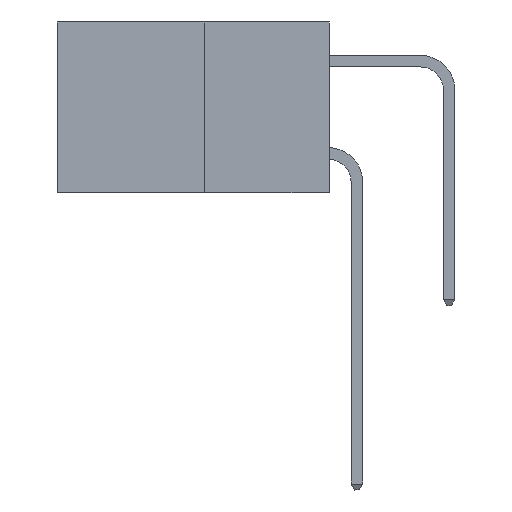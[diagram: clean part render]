
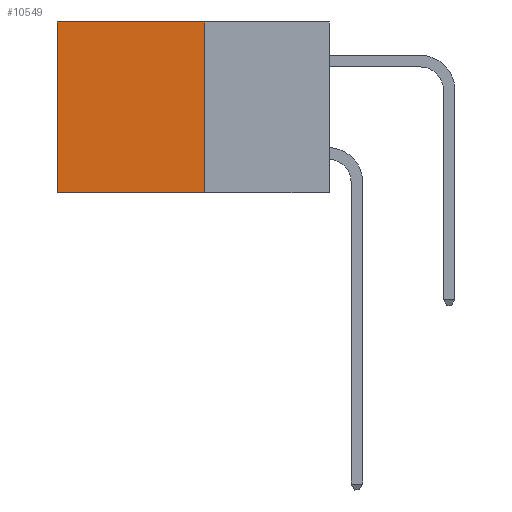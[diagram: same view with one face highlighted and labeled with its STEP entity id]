
A CAD part, left-side view. The second image highlights one B-rep face of the part: STEP entity #10549.
In plain terms, the highlighted planar face has unit normal (-1, 0, 0).
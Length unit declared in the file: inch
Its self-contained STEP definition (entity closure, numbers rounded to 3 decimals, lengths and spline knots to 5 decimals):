
#192 = AXIS2_PLACEMENT_3D ( 'NONE', #8386, #10762, #3405 ) ;
#1339 = DIRECTION ( 'NONE',  ( 0., 1., 0. ) ) ;
#1359 = ORIENTED_EDGE ( 'NONE', *, *, #1635, .T. ) ;
#1572 = CARTESIAN_POINT ( 'NONE',  ( 0.277, 0.27, -0.37 ) ) ;
#1635 = EDGE_CURVE ( 'NONE', #6401, #8254, #6325, .T. ) ;
#2506 = ORIENTED_EDGE ( 'NONE', *, *, #9012, .T. ) ;
#2577 = VECTOR ( 'NONE', #10705, 39.37008 ) ;
#3405 = DIRECTION ( 'NONE',  ( 0., 0., -1. ) ) ;
#3964 = VERTEX_POINT ( 'NONE', #10169 ) ;
#5584 = EDGE_CURVE ( 'NONE', #3964, #8254, #15202, .T. ) ;
#6325 = LINE ( 'NONE', #10808, #2577 ) ;
#6401 = VERTEX_POINT ( 'NONE', #11030 ) ;
#6973 = ORIENTED_EDGE ( 'NONE', *, *, #5584, .F. ) ;
#7156 = PLANE ( 'NONE',  #192 ) ;
#7294 = EDGE_CURVE ( 'NONE', #9734, #3964, #13034, .T. ) ;
#8116 = FACE_OUTER_BOUND ( 'NONE', #10496, .T. ) ;
#8254 = VERTEX_POINT ( 'NONE', #13641 ) ;
#8386 = CARTESIAN_POINT ( 'NONE',  ( 0.277, 0.27, -0.37 ) ) ;
#9012 = EDGE_CURVE ( 'NONE', #9734, #6401, #12447, .T. ) ;
#9734 = VERTEX_POINT ( 'NONE', #9985 ) ;
#9838 = DIRECTION ( 'NONE',  ( 0., 0., -1. ) ) ;
#9985 = CARTESIAN_POINT ( 'NONE',  ( 0.277, 0.27, 0. ) ) ;
#10169 = CARTESIAN_POINT ( 'NONE',  ( 0.277, 0.27, -0.37 ) ) ;
#10496 = EDGE_LOOP ( 'NONE', ( #1359, #6973, #11989, #2506 ) ) ;
#10549 = ADVANCED_FACE ( 'NONE', ( #8116 ), #7156, .F. ) ;
#10705 = DIRECTION ( 'NONE',  ( 0., 0., -1. ) ) ;
#10762 = DIRECTION ( 'NONE',  ( 1., 0., 0. ) ) ;
#10808 = CARTESIAN_POINT ( 'NONE',  ( 0.277, 0.59, -0.37 ) ) ;
#11030 = CARTESIAN_POINT ( 'NONE',  ( 0.277, 0.59, 0. ) ) ;
#11673 = DIRECTION ( 'NONE',  ( 0., 1., 0. ) ) ;
#11989 = ORIENTED_EDGE ( 'NONE', *, *, #7294, .F. ) ;
#12142 = VECTOR ( 'NONE', #11673, 39.37008 ) ;
#12447 = LINE ( 'NONE', #15809, #15136 ) ;
#13034 = LINE ( 'NONE', #15601, #13387 ) ;
#13387 = VECTOR ( 'NONE', #9838, 39.37008 ) ;
#13641 = CARTESIAN_POINT ( 'NONE',  ( 0.277, 0.59, -0.37 ) ) ;
#15136 = VECTOR ( 'NONE', #1339, 39.37008 ) ;
#15202 = LINE ( 'NONE', #1572, #12142 ) ;
#15601 = CARTESIAN_POINT ( 'NONE',  ( 0.277, 0.27, -0.37 ) ) ;
#15809 = CARTESIAN_POINT ( 'NONE',  ( 0.277, 0.27, 0. ) ) ;
